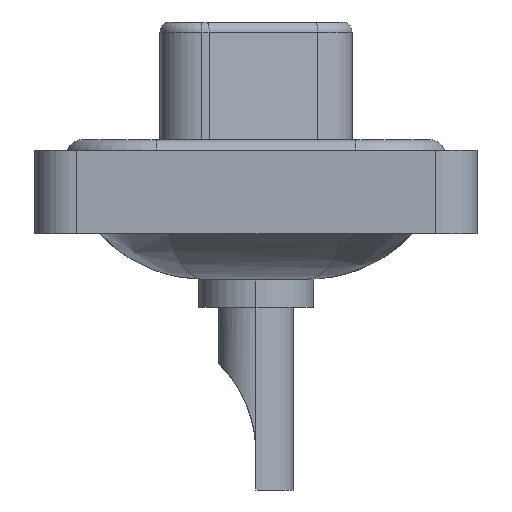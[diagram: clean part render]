
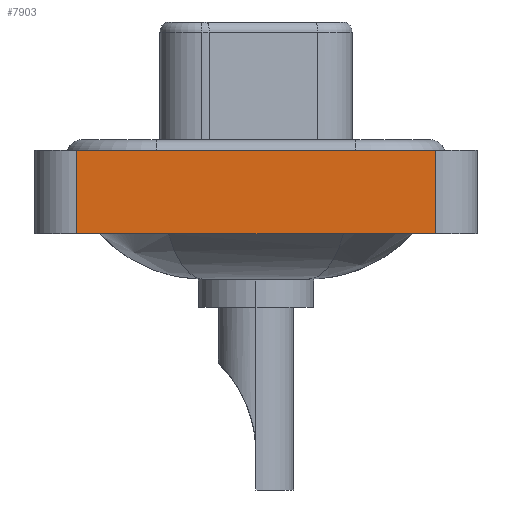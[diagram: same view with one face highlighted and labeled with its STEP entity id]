
A CAD part, left-side view. The second image highlights one B-rep face of the part: STEP entity #7903.
In plain terms, the highlighted planar face has unit normal (-1, 0, 0).
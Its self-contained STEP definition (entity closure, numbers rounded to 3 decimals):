
#466 = LINE ( 'NONE', #16810, #10825 ) ;
#1893 = ORIENTED_EDGE ( 'NONE', *, *, #17711, .F. ) ;
#2046 = VECTOR ( 'NONE', #14740, 1000. ) ;
#2095 = VECTOR ( 'NONE', #13553, 1000. ) ;
#2284 = EDGE_LOOP ( 'NONE', ( #18548, #12142, #1893, #5349 ) ) ;
#2371 = EDGE_CURVE ( 'NONE', #7638, #18904, #11894, .T. ) ;
#2631 = LINE ( 'NONE', #2829, #2095 ) ;
#2829 = CARTESIAN_POINT ( 'NONE',  ( -7.3, -8.55, -3.6 ) ) ;
#4001 = AXIS2_PLACEMENT_3D ( 'NONE', #7211, #14920, #13265 ) ;
#4030 = PLANE ( 'NONE',  #4001 ) ;
#5349 = ORIENTED_EDGE ( 'NONE', *, *, #2371, .T. ) ;
#5727 = FACE_OUTER_BOUND ( 'NONE', #2284, .T. ) ;
#6637 = CARTESIAN_POINT ( 'NONE',  ( -7.3, 8.55, -3.6 ) ) ;
#7211 = CARTESIAN_POINT ( 'NONE',  ( -7.3, -8.55, -3.6 ) ) ;
#7425 = VECTOR ( 'NONE', #8216, 1000. ) ;
#7638 = VERTEX_POINT ( 'NONE', #13960 ) ;
#7903 = ADVANCED_FACE ( 'NONE', ( #5727 ), #4030, .T. ) ;
#8216 = DIRECTION ( 'NONE',  ( 0., 0., 1. ) ) ;
#8812 = CARTESIAN_POINT ( 'NONE',  ( -7.3, -8.55, 0.4 ) ) ;
#9406 = VERTEX_POINT ( 'NONE', #8812 ) ;
#10825 = VECTOR ( 'NONE', #18204, 1000. ) ;
#11105 = LINE ( 'NONE', #6637, #7425 ) ;
#11878 = EDGE_CURVE ( 'NONE', #13624, #9406, #466, .T. ) ;
#11894 = LINE ( 'NONE', #11995, #2046 ) ;
#11995 = CARTESIAN_POINT ( 'NONE',  ( -7.3, -8.55, -3.6 ) ) ;
#12142 = ORIENTED_EDGE ( 'NONE', *, *, #11878, .F. ) ;
#12619 = EDGE_CURVE ( 'NONE', #18904, #9406, #2631, .T. ) ;
#13265 = DIRECTION ( 'NONE',  ( 0., 0., 1. ) ) ;
#13553 = DIRECTION ( 'NONE',  ( 0., 0., 1. ) ) ;
#13624 = VERTEX_POINT ( 'NONE', #14410 ) ;
#13960 = CARTESIAN_POINT ( 'NONE',  ( -7.3, 8.55, -3.6 ) ) ;
#14410 = CARTESIAN_POINT ( 'NONE',  ( -7.3, 8.55, 0.4 ) ) ;
#14740 = DIRECTION ( 'NONE',  ( 0., -1., 0. ) ) ;
#14920 = DIRECTION ( 'NONE',  ( -1., 0., 0. ) ) ;
#16810 = CARTESIAN_POINT ( 'NONE',  ( -7.3, -8.55, 0.4 ) ) ;
#17711 = EDGE_CURVE ( 'NONE', #7638, #13624, #11105, .T. ) ;
#18204 = DIRECTION ( 'NONE',  ( 0., -1., 0. ) ) ;
#18548 = ORIENTED_EDGE ( 'NONE', *, *, #12619, .T. ) ;
#18904 = VERTEX_POINT ( 'NONE', #19551 ) ;
#19551 = CARTESIAN_POINT ( 'NONE',  ( -7.3, -8.55, -3.6 ) ) ;
